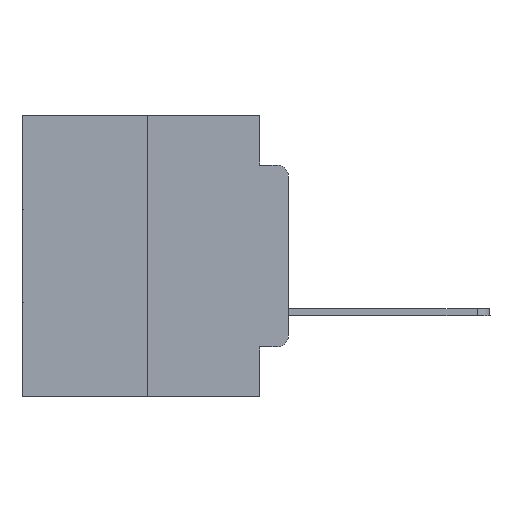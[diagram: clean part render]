
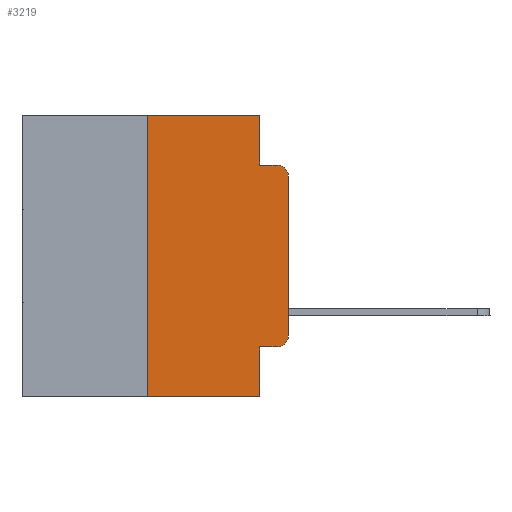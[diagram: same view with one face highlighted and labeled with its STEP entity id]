
A CAD part, left-side view. The second image highlights one B-rep face of the part: STEP entity #3219.
In plain terms, the highlighted planar face has unit normal (-1, 0, 0).
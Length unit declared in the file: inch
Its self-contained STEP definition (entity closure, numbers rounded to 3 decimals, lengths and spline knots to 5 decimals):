
#21 = EDGE_CURVE ( 'NONE', #18413, #27670, #10507, .T. ) ;
#175 = ORIENTED_EDGE ( 'NONE', *, *, #4686, .T. ) ;
#831 = FACE_OUTER_BOUND ( 'NONE', #9546, .T. ) ;
#1005 = VECTOR ( 'NONE', #10543, 39.37008 ) ;
#1145 = AXIS2_PLACEMENT_3D ( 'NONE', #18552, #1418, #18913 ) ;
#1302 = DIRECTION ( 'NONE',  ( 0., -1., 0. ) ) ;
#1418 = DIRECTION ( 'NONE',  ( -1., 0., 0. ) ) ;
#1431 = LINE ( 'NONE', #2817, #6587 ) ;
#1649 = VECTOR ( 'NONE', #17499, 39.37008 ) ;
#1681 = LINE ( 'NONE', #7666, #1005 ) ;
#1850 = VERTEX_POINT ( 'NONE', #9962 ) ;
#2194 = CARTESIAN_POINT ( 'NONE',  ( 0., 0.051, 0. ) ) ;
#2324 = CARTESIAN_POINT ( 'NONE',  ( 0., 0., 0. ) ) ;
#2645 = ORIENTED_EDGE ( 'NONE', *, *, #26050, .F. ) ;
#2659 = CARTESIAN_POINT ( 'NONE',  ( 0., 0.02, -0.4115 ) ) ;
#2817 = CARTESIAN_POINT ( 'NONE',  ( 0., 0.473, -0.5 ) ) ;
#3183 = LINE ( 'NONE', #26024, #14486 ) ;
#3210 = CARTESIAN_POINT ( 'NONE',  ( 0., 0.051, -0.4115 ) ) ;
#3219 = ADVANCED_FACE ( 'NONE', ( #831 ), #17679, .F. ) ;
#3379 = AXIS2_PLACEMENT_3D ( 'NONE', #7797, #16221, #9741 ) ;
#3605 = EDGE_CURVE ( 'NONE', #27670, #20028, #23751, .T. ) ;
#3909 = CARTESIAN_POINT ( 'NONE',  ( 0., 0.051, 0. ) ) ;
#4068 = CARTESIAN_POINT ( 'NONE',  ( 0., 0.051, -0.5 ) ) ;
#4686 = EDGE_CURVE ( 'NONE', #15206, #26493, #1431, .T. ) ;
#4758 = EDGE_CURVE ( 'NONE', #17853, #5335, #22304, .T. ) ;
#4923 = DIRECTION ( 'NONE',  ( 0., 0., 1. ) ) ;
#5245 = CARTESIAN_POINT ( 'NONE',  ( 0., 0.02, -0.0885 ) ) ;
#5335 = VERTEX_POINT ( 'NONE', #5245 ) ;
#5469 = CARTESIAN_POINT ( 'NONE',  ( 0., 0., -0.1085 ) ) ;
#5701 = VECTOR ( 'NONE', #7803, 39.37008 ) ;
#5995 = LINE ( 'NONE', #27417, #22079 ) ;
#6113 = DIRECTION ( 'NONE',  ( 0., 0., -1. ) ) ;
#6587 = VECTOR ( 'NONE', #9620, 39.37008 ) ;
#6769 = ORIENTED_EDGE ( 'NONE', *, *, #3605, .T. ) ;
#6772 = CARTESIAN_POINT ( 'NONE',  ( 0., 0.473, 0. ) ) ;
#7666 = CARTESIAN_POINT ( 'NONE',  ( 0., 0.051, -0.0885 ) ) ;
#7797 = CARTESIAN_POINT ( 'NONE',  ( 0., 0.02, -0.1085 ) ) ;
#7803 = DIRECTION ( 'NONE',  ( 0., -1., 0. ) ) ;
#8220 = CARTESIAN_POINT ( 'NONE',  ( 0., 0.25, 0. ) ) ;
#9376 = ORIENTED_EDGE ( 'NONE', *, *, #27017, .F. ) ;
#9546 = EDGE_LOOP ( 'NONE', ( #21615, #19213, #21452, #2645, #11190, #19176, #175, #9376, #18027, #6769 ) ) ;
#9620 = DIRECTION ( 'NONE',  ( 0., -1., 0. ) ) ;
#9633 = VECTOR ( 'NONE', #6113, 39.37008 ) ;
#9715 = CARTESIAN_POINT ( 'NONE',  ( 0., 0.25, -0.5 ) ) ;
#9741 = DIRECTION ( 'NONE',  ( 0., 0., -1. ) ) ;
#9962 = CARTESIAN_POINT ( 'NONE',  ( 0., 0.051, 0. ) ) ;
#9973 = CARTESIAN_POINT ( 'NONE',  ( 0., 0.051, -0.4115 ) ) ;
#10507 = LINE ( 'NONE', #3210, #5701 ) ;
#10543 = DIRECTION ( 'NONE',  ( 0., -1., 0. ) ) ;
#10980 = VECTOR ( 'NONE', #4923, 39.37008 ) ;
#11190 = ORIENTED_EDGE ( 'NONE', *, *, #16051, .F. ) ;
#12391 = EDGE_CURVE ( 'NONE', #15864, #5335, #1681, .T. ) ;
#12914 = DIRECTION ( 'NONE',  ( 0., 0., 1. ) ) ;
#14030 = LINE ( 'NONE', #2324, #10980 ) ;
#14486 = VECTOR ( 'NONE', #12914, 39.37008 ) ;
#15206 = VERTEX_POINT ( 'NONE', #9715 ) ;
#15864 = VERTEX_POINT ( 'NONE', #21346 ) ;
#16051 = EDGE_CURVE ( 'NONE', #19277, #1850, #5995, .T. ) ;
#16221 = DIRECTION ( 'NONE',  ( -1., 0., 0. ) ) ;
#16790 = LINE ( 'NONE', #3909, #9633 ) ;
#17464 = CARTESIAN_POINT ( 'NONE',  ( 0., 0., -0.3915 ) ) ;
#17499 = DIRECTION ( 'NONE',  ( 0., 0., -1. ) ) ;
#17589 = DIRECTION ( 'NONE',  ( 0., 0., -1. ) ) ;
#17679 = PLANE ( 'NONE',  #21854 ) ;
#17853 = VERTEX_POINT ( 'NONE', #5469 ) ;
#18027 = ORIENTED_EDGE ( 'NONE', *, *, #21, .T. ) ;
#18413 = VERTEX_POINT ( 'NONE', #9973 ) ;
#18552 = CARTESIAN_POINT ( 'NONE',  ( 0., 0.02, -0.3915 ) ) ;
#18913 = DIRECTION ( 'NONE',  ( 0., 0., -1. ) ) ;
#19176 = ORIENTED_EDGE ( 'NONE', *, *, #19498, .F. ) ;
#19213 = ORIENTED_EDGE ( 'NONE', *, *, #4758, .T. ) ;
#19277 = VERTEX_POINT ( 'NONE', #8220 ) ;
#19498 = EDGE_CURVE ( 'NONE', #15206, #19277, #3183, .T. ) ;
#20028 = VERTEX_POINT ( 'NONE', #17464 ) ;
#21158 = EDGE_CURVE ( 'NONE', #20028, #17853, #14030, .T. ) ;
#21346 = CARTESIAN_POINT ( 'NONE',  ( 0., 0.051, -0.0885 ) ) ;
#21452 = ORIENTED_EDGE ( 'NONE', *, *, #12391, .F. ) ;
#21615 = ORIENTED_EDGE ( 'NONE', *, *, #21158, .T. ) ;
#21854 = AXIS2_PLACEMENT_3D ( 'NONE', #6772, #26200, #17589 ) ;
#22079 = VECTOR ( 'NONE', #1302, 39.37008 ) ;
#22304 = CIRCLE ( 'NONE', #3379, 0.02 ) ;
#23751 = CIRCLE ( 'NONE', #1145, 0.02 ) ;
#26024 = CARTESIAN_POINT ( 'NONE',  ( 0., 0.25, 0. ) ) ;
#26050 = EDGE_CURVE ( 'NONE', #1850, #15864, #16790, .T. ) ;
#26200 = DIRECTION ( 'NONE',  ( 1., 0., 0. ) ) ;
#26321 = LINE ( 'NONE', #2194, #1649 ) ;
#26493 = VERTEX_POINT ( 'NONE', #4068 ) ;
#27017 = EDGE_CURVE ( 'NONE', #18413, #26493, #26321, .T. ) ;
#27417 = CARTESIAN_POINT ( 'NONE',  ( 0., 0.473, 0. ) ) ;
#27670 = VERTEX_POINT ( 'NONE', #2659 ) ;
